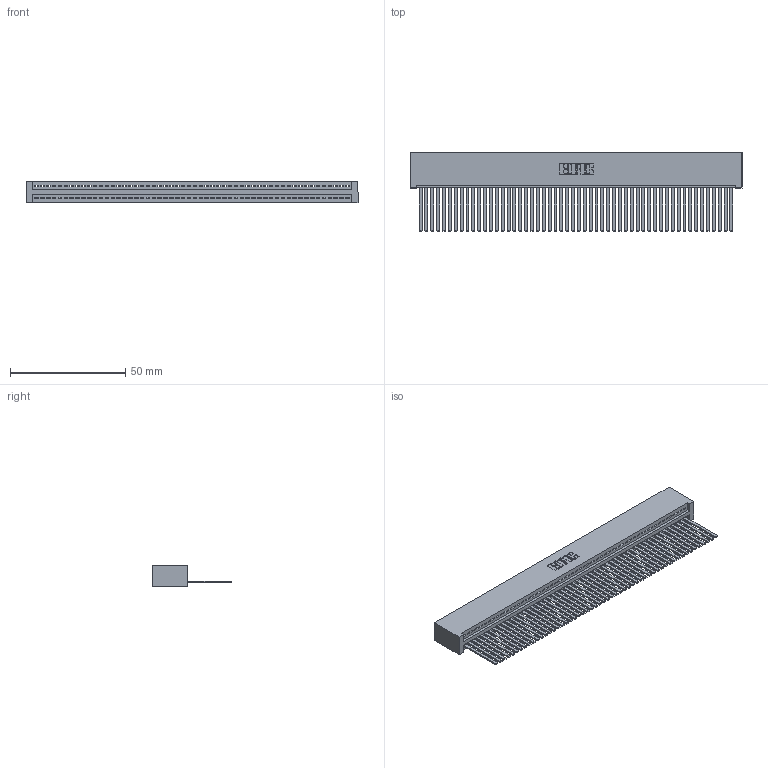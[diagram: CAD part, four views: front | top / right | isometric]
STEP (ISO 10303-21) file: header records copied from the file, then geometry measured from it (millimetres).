
FILE_DESCRIPTION (( 'STEP AP203' ), '1' );
FILE_NAME ('345-054-544-101.STEP', '2019-10-10T00:40:12', ( '' ), ( '' ), 'SwSTEP 2.0', 'SolidWorks 2016', '' );
FILE_SCHEMA (( 'CONFIG_CONTROL_DESIGN' ));
Length unit declared in the file: inch
Products named in the file (3): 345 Part_No Mounting Lugs; 345-054-544-101; 345-292-001_345-293-144
Assembly tree (55 placements, depth 2):
  345-054-544-101
    345 Part_No Mounting Lugs
    345-292-001_345-293-144  x54
Bounding box: 143.76 x 33.96 x 9.4 mm (x, y, z)
Volume: 14962.9 mm3; surface area: 22115.1 mm2
Topology: 55 solids, 55 shells, 2926 faces, 8849 edges, 5826 vertices
Faces by surface type: plane 2020, cylinder 906
Entity records: 38565 total; most frequent: CARTESIAN_POINT 6686, ORIENTED_EDGE 6674, DIRECTION 5813, EDGE_CURVE 3337, LINE 3001, VECTOR 3001, VERTEX_POINT 2222, AXIS2_PLACEMENT_3D 1406
